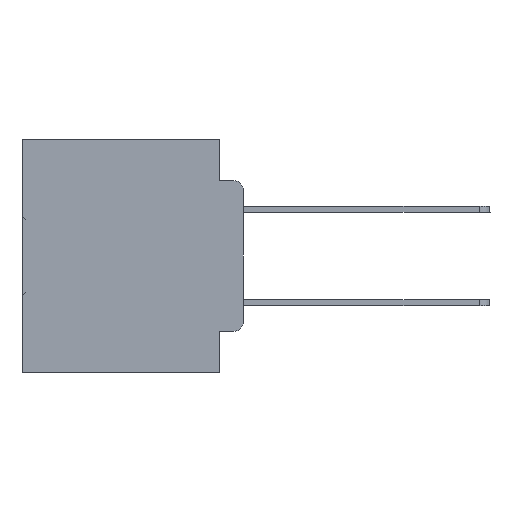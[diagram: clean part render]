
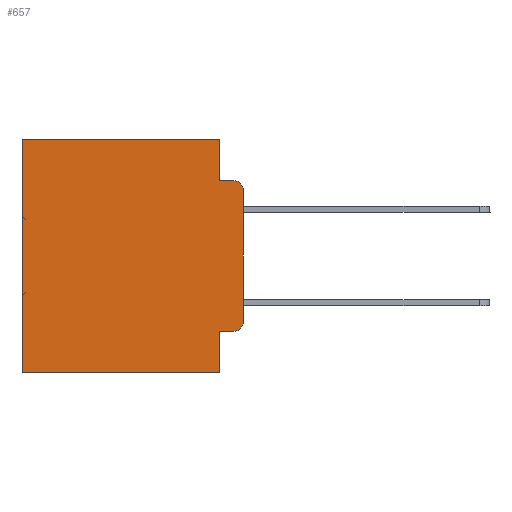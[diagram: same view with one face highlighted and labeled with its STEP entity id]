
A CAD part, left-side view. The second image highlights one B-rep face of the part: STEP entity #657.
In plain terms, the highlighted planar face has unit normal (-1, 0, 0).
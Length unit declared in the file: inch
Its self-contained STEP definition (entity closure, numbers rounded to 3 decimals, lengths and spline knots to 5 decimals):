
#238 = DIRECTION ( 'NONE',  ( 0., -1., 0. ) ) ;
#657 = ADVANCED_FACE ( 'NONE', ( #24782 ), #15811, .F. ) ;
#1275 = VECTOR ( 'NONE', #19187, 39.37008 ) ;
#3244 = VECTOR ( 'NONE', #5505, 39.37008 ) ;
#3339 = AXIS2_PLACEMENT_3D ( 'NONE', #28987, #31574, #32113 ) ;
#3574 = LINE ( 'NONE', #22838, #22268 ) ;
#3897 = VERTEX_POINT ( 'NONE', #18233 ) ;
#4070 = CARTESIAN_POINT ( 'NONE',  ( 0.298, 0.051, 0. ) ) ;
#4800 = DIRECTION ( 'NONE',  ( 0., 0., -1. ) ) ;
#4835 = VECTOR ( 'NONE', #25727, 39.37008 ) ;
#5505 = DIRECTION ( 'NONE',  ( 0., 0., -1. ) ) ;
#5687 = ORIENTED_EDGE ( 'NONE', *, *, #12253, .T. ) ;
#5697 = CARTESIAN_POINT ( 'NONE',  ( 0.298, 0., 0. ) ) ;
#5810 = ORIENTED_EDGE ( 'NONE', *, *, #16557, .F. ) ;
#6654 = CARTESIAN_POINT ( 'NONE',  ( 0.298, 0.051, 0. ) ) ;
#7162 = ORIENTED_EDGE ( 'NONE', *, *, #33612, .T. ) ;
#7365 = ORIENTED_EDGE ( 'NONE', *, *, #29982, .F. ) ;
#7516 = CARTESIAN_POINT ( 'NONE',  ( 0.298, 0.02, -0.1085 ) ) ;
#7706 = CARTESIAN_POINT ( 'NONE',  ( 0.298, 0.051, 0. ) ) ;
#10650 = DIRECTION ( 'NONE',  ( 0., 0., -1. ) ) ;
#11223 = CARTESIAN_POINT ( 'NONE',  ( 0.298, 0.473, 0. ) ) ;
#11503 = EDGE_CURVE ( 'NONE', #12011, #22597, #12248, .T. ) ;
#11534 = LINE ( 'NONE', #30443, #26163 ) ;
#12011 = VERTEX_POINT ( 'NONE', #27620 ) ;
#12248 = CIRCLE ( 'NONE', #18681, 0.02 ) ;
#12253 = EDGE_CURVE ( 'NONE', #26189, #22137, #3574, .T. ) ;
#12726 = CIRCLE ( 'NONE', #3339, 0.02 ) ;
#15509 = VECTOR ( 'NONE', #4800, 39.37008 ) ;
#15811 = PLANE ( 'NONE',  #28665 ) ;
#15954 = LINE ( 'NONE', #7706, #35339 ) ;
#16557 = EDGE_CURVE ( 'NONE', #31303, #22597, #22477, .T. ) ;
#18025 = LINE ( 'NONE', #4070, #15509 ) ;
#18233 = CARTESIAN_POINT ( 'NONE',  ( 0.298, 0.051, -0.5 ) ) ;
#18681 = AXIS2_PLACEMENT_3D ( 'NONE', #7516, #32106, #24561 ) ;
#18784 = EDGE_CURVE ( 'NONE', #29643, #31303, #18025, .T. ) ;
#18911 = DIRECTION ( 'NONE',  ( 1., 0., 0. ) ) ;
#19187 = DIRECTION ( 'NONE',  ( 0., -1., 0. ) ) ;
#19454 = LINE ( 'NONE', #5697, #3244 ) ;
#19532 = EDGE_LOOP ( 'NONE', ( #30045, #20339, #5810, #24076, #25133, #7162, #7365, #36147, #5687, #23741 ) ) ;
#20024 = LINE ( 'NONE', #28671, #4835 ) ;
#20339 = ORIENTED_EDGE ( 'NONE', *, *, #11503, .T. ) ;
#20534 = VECTOR ( 'NONE', #32455, 39.37008 ) ;
#21250 = CARTESIAN_POINT ( 'NONE',  ( 0.298, 0.473, 0. ) ) ;
#21557 = VERTEX_POINT ( 'NONE', #24846 ) ;
#22137 = VERTEX_POINT ( 'NONE', #34290 ) ;
#22268 = VECTOR ( 'NONE', #238, 39.37008 ) ;
#22477 = LINE ( 'NONE', #33143, #1275 ) ;
#22591 = CARTESIAN_POINT ( 'NONE',  ( 0.298, 0.473, -0.5 ) ) ;
#22597 = VERTEX_POINT ( 'NONE', #34066 ) ;
#22838 = CARTESIAN_POINT ( 'NONE',  ( 0.298, 0.051, -0.4115 ) ) ;
#23741 = ORIENTED_EDGE ( 'NONE', *, *, #28380, .T. ) ;
#24001 = LINE ( 'NONE', #21250, #20534 ) ;
#24076 = ORIENTED_EDGE ( 'NONE', *, *, #18784, .F. ) ;
#24254 = CARTESIAN_POINT ( 'NONE',  ( 0.298, 0.051, -0.0885 ) ) ;
#24561 = DIRECTION ( 'NONE',  ( 0., 0., -1. ) ) ;
#24608 = DIRECTION ( 'NONE',  ( 0., 0., -1. ) ) ;
#24618 = EDGE_CURVE ( 'NONE', #26189, #3897, #15954, .T. ) ;
#24782 = FACE_OUTER_BOUND ( 'NONE', #19532, .T. ) ;
#24846 = CARTESIAN_POINT ( 'NONE',  ( 0.298, 0., -0.3915 ) ) ;
#24931 = DIRECTION ( 'NONE',  ( 0., 1., 0. ) ) ;
#25133 = ORIENTED_EDGE ( 'NONE', *, *, #34741, .T. ) ;
#25648 = VERTEX_POINT ( 'NONE', #22591 ) ;
#25727 = DIRECTION ( 'NONE',  ( 0., 1., 0. ) ) ;
#26163 = VECTOR ( 'NONE', #24931, 39.37008 ) ;
#26189 = VERTEX_POINT ( 'NONE', #26547 ) ;
#26547 = CARTESIAN_POINT ( 'NONE',  ( 0.298, 0.051, -0.4115 ) ) ;
#27620 = CARTESIAN_POINT ( 'NONE',  ( 0.298, 0., -0.1085 ) ) ;
#28320 = EDGE_CURVE ( 'NONE', #12011, #21557, #19454, .T. ) ;
#28380 = EDGE_CURVE ( 'NONE', #22137, #21557, #12726, .T. ) ;
#28665 = AXIS2_PLACEMENT_3D ( 'NONE', #35974, #18911, #24608 ) ;
#28671 = CARTESIAN_POINT ( 'NONE',  ( 0.298, 0., 0. ) ) ;
#28987 = CARTESIAN_POINT ( 'NONE',  ( 0.298, 0.02, -0.3915 ) ) ;
#29643 = VERTEX_POINT ( 'NONE', #6654 ) ;
#29982 = EDGE_CURVE ( 'NONE', #3897, #25648, #11534, .T. ) ;
#30045 = ORIENTED_EDGE ( 'NONE', *, *, #28320, .F. ) ;
#30443 = CARTESIAN_POINT ( 'NONE',  ( 0.298, 0., -0.5 ) ) ;
#31303 = VERTEX_POINT ( 'NONE', #24254 ) ;
#31574 = DIRECTION ( 'NONE',  ( -1., 0., 0. ) ) ;
#32106 = DIRECTION ( 'NONE',  ( -1., 0., 0. ) ) ;
#32113 = DIRECTION ( 'NONE',  ( 0., 0., -1. ) ) ;
#32455 = DIRECTION ( 'NONE',  ( 0., 0., -1. ) ) ;
#33143 = CARTESIAN_POINT ( 'NONE',  ( 0.298, 0.051, -0.0885 ) ) ;
#33612 = EDGE_CURVE ( 'NONE', #35670, #25648, #24001, .T. ) ;
#34066 = CARTESIAN_POINT ( 'NONE',  ( 0.298, 0.02, -0.0885 ) ) ;
#34290 = CARTESIAN_POINT ( 'NONE',  ( 0.298, 0.02, -0.4115 ) ) ;
#34741 = EDGE_CURVE ( 'NONE', #29643, #35670, #20024, .T. ) ;
#35339 = VECTOR ( 'NONE', #10650, 39.37008 ) ;
#35670 = VERTEX_POINT ( 'NONE', #11223 ) ;
#35974 = CARTESIAN_POINT ( 'NONE',  ( 0.298, 0., 0. ) ) ;
#36147 = ORIENTED_EDGE ( 'NONE', *, *, #24618, .F. ) ;
